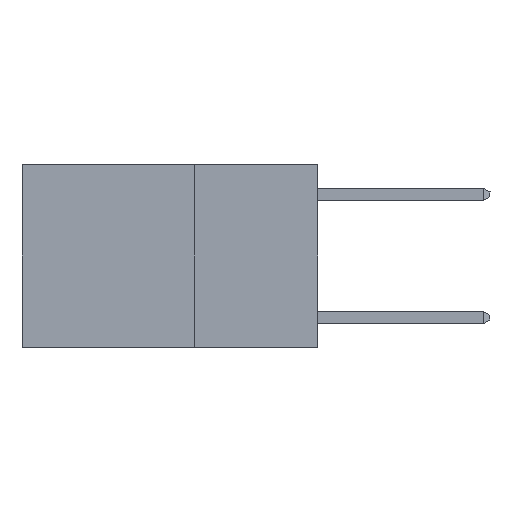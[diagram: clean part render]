
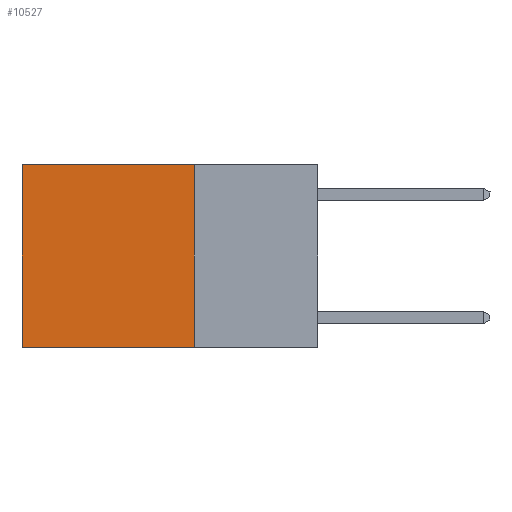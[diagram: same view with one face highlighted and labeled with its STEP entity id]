
A CAD part, left-side view. The second image highlights one B-rep face of the part: STEP entity #10527.
In plain terms, the highlighted planar face has unit normal (-1, 0, 0).
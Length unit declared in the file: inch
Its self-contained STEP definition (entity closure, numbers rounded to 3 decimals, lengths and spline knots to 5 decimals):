
#1335 = EDGE_CURVE ( 'NONE', #1983, #6233, #8322, .T. ) ;
#1983 = VERTEX_POINT ( 'NONE', #10110 ) ;
#3376 = EDGE_LOOP ( 'NONE', ( #7350, #11489, #7010, #12232 ) ) ;
#3974 = EDGE_CURVE ( 'NONE', #14042, #6233, #13431, .T. ) ;
#4075 = VECTOR ( 'NONE', #11379, 39.37008 ) ;
#4578 = CARTESIAN_POINT ( 'NONE',  ( 0.2625, 0.6, 0. ) ) ;
#4600 = CARTESIAN_POINT ( 'NONE',  ( 0.2625, 0.25, 0. ) ) ;
#4815 = CARTESIAN_POINT ( 'NONE',  ( 0.2625, 0.25, 0. ) ) ;
#5396 = AXIS2_PLACEMENT_3D ( 'NONE', #10886, #14213, #7580 ) ;
#6046 = LINE ( 'NONE', #4815, #12002 ) ;
#6233 = VERTEX_POINT ( 'NONE', #11161 ) ;
#6510 = EDGE_CURVE ( 'NONE', #7612, #1983, #6046, .T. ) ;
#6641 = CARTESIAN_POINT ( 'NONE',  ( 0.2625, 0.25, 0. ) ) ;
#7010 = ORIENTED_EDGE ( 'NONE', *, *, #6510, .F. ) ;
#7350 = ORIENTED_EDGE ( 'NONE', *, *, #3974, .T. ) ;
#7526 = PLANE ( 'NONE',  #5396 ) ;
#7532 = VECTOR ( 'NONE', #8012, 39.37008 ) ;
#7580 = DIRECTION ( 'NONE',  ( 0., 0., -1. ) ) ;
#7612 = VERTEX_POINT ( 'NONE', #6641 ) ;
#8012 = DIRECTION ( 'NONE',  ( 0., 0., -1. ) ) ;
#8322 = LINE ( 'NONE', #10095, #13859 ) ;
#8671 = DIRECTION ( 'NONE',  ( 0., 1., 0. ) ) ;
#9358 = DIRECTION ( 'NONE',  ( 0., 0., -1. ) ) ;
#10095 = CARTESIAN_POINT ( 'NONE',  ( 0.2625, 0.25, -0.37 ) ) ;
#10110 = CARTESIAN_POINT ( 'NONE',  ( 0.2625, 0.25, -0.37 ) ) ;
#10140 = EDGE_CURVE ( 'NONE', #7612, #14042, #10413, .T. ) ;
#10413 = LINE ( 'NONE', #4600, #4075 ) ;
#10527 = ADVANCED_FACE ( 'NONE', ( #13704 ), #7526, .F. ) ;
#10886 = CARTESIAN_POINT ( 'NONE',  ( 0.2625, 0.25, 0. ) ) ;
#11161 = CARTESIAN_POINT ( 'NONE',  ( 0.2625, 0.6, -0.37 ) ) ;
#11379 = DIRECTION ( 'NONE',  ( 0., 1., 0. ) ) ;
#11489 = ORIENTED_EDGE ( 'NONE', *, *, #1335, .F. ) ;
#11734 = CARTESIAN_POINT ( 'NONE',  ( 0.2625, 0.6, 0. ) ) ;
#12002 = VECTOR ( 'NONE', #9358, 39.37008 ) ;
#12232 = ORIENTED_EDGE ( 'NONE', *, *, #10140, .T. ) ;
#13431 = LINE ( 'NONE', #4578, #7532 ) ;
#13704 = FACE_OUTER_BOUND ( 'NONE', #3376, .T. ) ;
#13859 = VECTOR ( 'NONE', #8671, 39.37008 ) ;
#14042 = VERTEX_POINT ( 'NONE', #11734 ) ;
#14213 = DIRECTION ( 'NONE',  ( 1., 0., 0. ) ) ;
